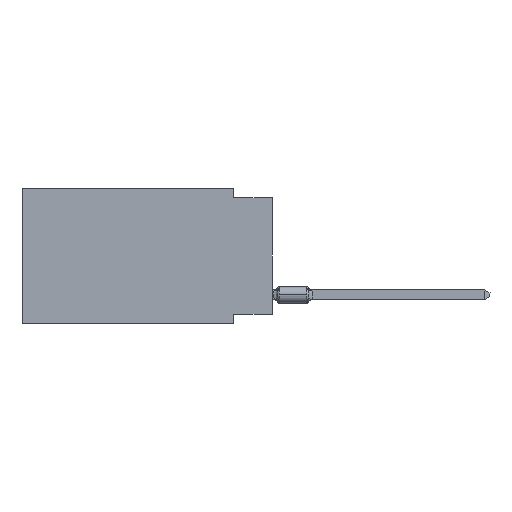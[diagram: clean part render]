
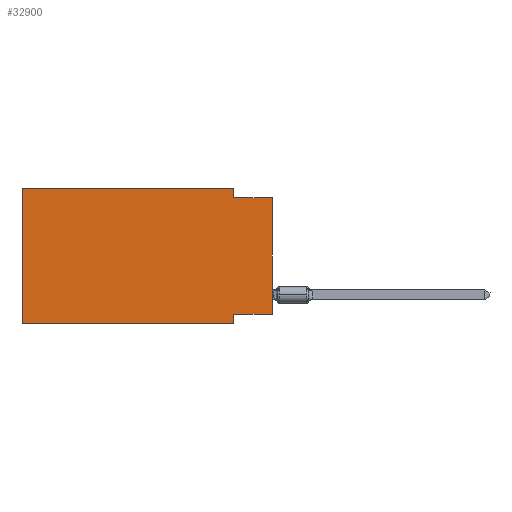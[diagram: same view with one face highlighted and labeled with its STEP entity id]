
A CAD part, left-side view. The second image highlights one B-rep face of the part: STEP entity #32900.
In plain terms, the highlighted planar face has unit normal (-1, 0, 0).
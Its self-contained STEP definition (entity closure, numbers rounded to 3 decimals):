
#875 = CARTESIAN_POINT ( 'NONE',  ( 0., 16.383, 0. ) ) ;
#1296 = CARTESIAN_POINT ( 'NONE',  ( 0., 16.383, -8.89 ) ) ;
#1363 = VERTEX_POINT ( 'NONE', #1296 ) ;
#2327 = LINE ( 'NONE', #24897, #11521 ) ;
#3323 = LINE ( 'NONE', #13519, #32890 ) ;
#3368 = ORIENTED_EDGE ( 'NONE', *, *, #32929, .T. ) ;
#3380 = DIRECTION ( 'NONE',  ( 0., 0., -1. ) ) ;
#3437 = ORIENTED_EDGE ( 'NONE', *, *, #7779, .T. ) ;
#3722 = VERTEX_POINT ( 'NONE', #6903 ) ;
#4895 = EDGE_CURVE ( 'NONE', #13082, #29306, #3323, .T. ) ;
#5189 = ORIENTED_EDGE ( 'NONE', *, *, #9613, .F. ) ;
#6802 = CARTESIAN_POINT ( 'NONE',  ( 0., 16.383, 0. ) ) ;
#6903 = CARTESIAN_POINT ( 'NONE',  ( 0., 2.54, -8.89 ) ) ;
#7195 = DIRECTION ( 'NONE',  ( 0., 0., -1. ) ) ;
#7393 = ORIENTED_EDGE ( 'NONE', *, *, #7981, .F. ) ;
#7779 = EDGE_CURVE ( 'NONE', #1363, #3722, #22856, .T. ) ;
#7852 = CARTESIAN_POINT ( 'NONE',  ( 0., 2.54, -8.255 ) ) ;
#7981 = EDGE_CURVE ( 'NONE', #21456, #15109, #19965, .T. ) ;
#8304 = CARTESIAN_POINT ( 'NONE',  ( 0., 2.54, 0. ) ) ;
#8320 = DIRECTION ( 'NONE',  ( 0., -1., 0. ) ) ;
#8395 = DIRECTION ( 'NONE',  ( 1., 0., 0. ) ) ;
#9032 = DIRECTION ( 'NONE',  ( 0., 0., 1. ) ) ;
#9528 = VERTEX_POINT ( 'NONE', #21431 ) ;
#9613 = EDGE_CURVE ( 'NONE', #15109, #9528, #2327, .T. ) ;
#10004 = CARTESIAN_POINT ( 'NONE',  ( 0., 2.54, -8.89 ) ) ;
#11521 = VECTOR ( 'NONE', #7195, 1000. ) ;
#11661 = DIRECTION ( 'NONE',  ( 0., -1., 0. ) ) ;
#12028 = CARTESIAN_POINT ( 'NONE',  ( 0., 0., -0.635 ) ) ;
#12509 = ORIENTED_EDGE ( 'NONE', *, *, #28942, .F. ) ;
#12669 = DIRECTION ( 'NONE',  ( 0., 0., -1. ) ) ;
#12676 = CARTESIAN_POINT ( 'NONE',  ( 0., 16.383, 0. ) ) ;
#12849 = ORIENTED_EDGE ( 'NONE', *, *, #15982, .F. ) ;
#13082 = VERTEX_POINT ( 'NONE', #20218 ) ;
#13234 = LINE ( 'NONE', #16243, #16799 ) ;
#13519 = CARTESIAN_POINT ( 'NONE',  ( 0., 0., -8.255 ) ) ;
#15109 = VERTEX_POINT ( 'NONE', #8304 ) ;
#15982 = EDGE_CURVE ( 'NONE', #1363, #21456, #26222, .T. ) ;
#16075 = FACE_OUTER_BOUND ( 'NONE', #28343, .T. ) ;
#16243 = CARTESIAN_POINT ( 'NONE',  ( 0., 0., 0. ) ) ;
#16579 = PLANE ( 'NONE',  #32771 ) ;
#16799 = VECTOR ( 'NONE', #26264, 1000. ) ;
#16877 = CARTESIAN_POINT ( 'NONE',  ( 0., 0., -0.635 ) ) ;
#17396 = VECTOR ( 'NONE', #12669, 1000. ) ;
#17542 = ORIENTED_EDGE ( 'NONE', *, *, #22212, .F. ) ;
#18052 = VECTOR ( 'NONE', #11661, 1000. ) ;
#18699 = CARTESIAN_POINT ( 'NONE',  ( 0., 16.383, 0. ) ) ;
#19965 = LINE ( 'NONE', #6802, #18052 ) ;
#20218 = CARTESIAN_POINT ( 'NONE',  ( 0., 0., -8.255 ) ) ;
#20342 = CARTESIAN_POINT ( 'NONE',  ( 0., 16.383, -8.89 ) ) ;
#20707 = VECTOR ( 'NONE', #8320, 1000. ) ;
#21431 = CARTESIAN_POINT ( 'NONE',  ( 0., 2.54, -0.635 ) ) ;
#21456 = VERTEX_POINT ( 'NONE', #12676 ) ;
#22212 = EDGE_CURVE ( 'NONE', #9528, #27914, #24395, .T. ) ;
#22213 = DIRECTION ( 'NONE',  ( 0., -1., 0. ) ) ;
#22692 = ORIENTED_EDGE ( 'NONE', *, *, #4895, .F. ) ;
#22856 = LINE ( 'NONE', #20342, #20707 ) ;
#23701 = DIRECTION ( 'NONE',  ( 0., 1., 0. ) ) ;
#24395 = LINE ( 'NONE', #12028, #30201 ) ;
#24897 = CARTESIAN_POINT ( 'NONE',  ( 0., 2.54, 0. ) ) ;
#26222 = LINE ( 'NONE', #18699, #27622 ) ;
#26264 = DIRECTION ( 'NONE',  ( 0., 0., 1. ) ) ;
#27622 = VECTOR ( 'NONE', #9032, 1000. ) ;
#27914 = VERTEX_POINT ( 'NONE', #16877 ) ;
#28209 = LINE ( 'NONE', #10004, #17396 ) ;
#28343 = EDGE_LOOP ( 'NONE', ( #3368, #17542, #5189, #7393, #12849, #3437, #12509, #22692 ) ) ;
#28942 = EDGE_CURVE ( 'NONE', #29306, #3722, #28209, .T. ) ;
#29306 = VERTEX_POINT ( 'NONE', #7852 ) ;
#30201 = VECTOR ( 'NONE', #22213, 1000. ) ;
#32771 = AXIS2_PLACEMENT_3D ( 'NONE', #875, #8395, #3380 ) ;
#32890 = VECTOR ( 'NONE', #23701, 1000. ) ;
#32900 = ADVANCED_FACE ( 'NONE', ( #16075 ), #16579, .F. ) ;
#32929 = EDGE_CURVE ( 'NONE', #13082, #27914, #13234, .T. ) ;
